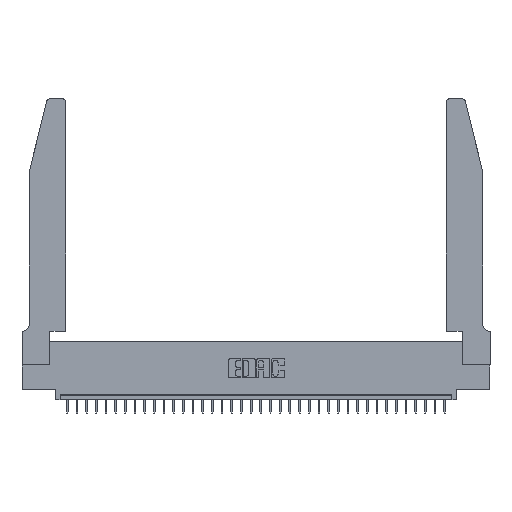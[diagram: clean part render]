
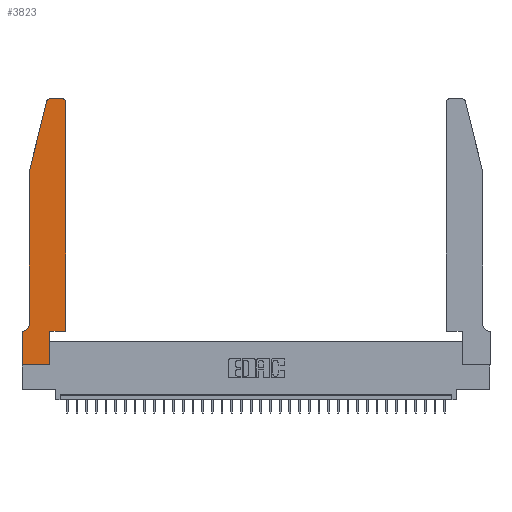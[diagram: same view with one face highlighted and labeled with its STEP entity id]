
A CAD part, top view. The second image highlights one B-rep face of the part: STEP entity #3823.
In plain terms, the highlighted planar face has unit normal (0, 0, 1).
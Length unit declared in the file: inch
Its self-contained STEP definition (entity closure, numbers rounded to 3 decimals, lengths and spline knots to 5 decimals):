
#847 = CARTESIAN_POINT ( 'NONE',  ( 0.25487, 2.72718, 0.37 ) ) ;
#1015 = ORIENTED_EDGE ( 'NONE', *, *, #24812, .T. ) ;
#1190 = ORIENTED_EDGE ( 'NONE', *, *, #3828, .T. ) ;
#1593 = DIRECTION ( 'NONE',  ( -1., 0., 0. ) ) ;
#1692 = VECTOR ( 'NONE', #20781, 39.37008 ) ;
#1829 = VERTEX_POINT ( 'NONE', #27603 ) ;
#2235 = CARTESIAN_POINT ( 'NONE',  ( 0.2865, 0., 0.37 ) ) ;
#2240 = DIRECTION ( 'NONE',  ( -0.239, -0.971, 0. ) ) ;
#2450 = CARTESIAN_POINT ( 'NONE',  ( 0.0755, 2., 0.37 ) ) ;
#3590 = LINE ( 'NONE', #11476, #9522 ) ;
#3823 = ADVANCED_FACE ( 'NONE', ( #34848 ), #24160, .T. ) ;
#3828 = EDGE_CURVE ( 'NONE', #14157, #1829, #30691, .T. ) ;
#3965 = CARTESIAN_POINT ( 'NONE',  ( 0.4505, 0.35, 0.37 ) ) ;
#4563 = VERTEX_POINT ( 'NONE', #3965 ) ;
#5346 = VERTEX_POINT ( 'NONE', #847 ) ;
#5575 = CARTESIAN_POINT ( 'NONE',  ( 0.2605, 2.75, 0.37 ) ) ;
#5810 = VERTEX_POINT ( 'NONE', #10276 ) ;
#6458 = DIRECTION ( 'NONE',  ( 0., 1., 0. ) ) ;
#6768 = CARTESIAN_POINT ( 'NONE',  ( 0., 0., 0.37 ) ) ;
#7005 = DIRECTION ( 'NONE',  ( 1., 0., 0. ) ) ;
#7046 = DIRECTION ( 'NONE',  ( 0., 0., 1. ) ) ;
#7713 = CARTESIAN_POINT ( 'NONE',  ( 0.0755, 0.42, 0.37 ) ) ;
#7977 = EDGE_CURVE ( 'NONE', #1829, #10247, #18263, .T. ) ;
#8146 = CARTESIAN_POINT ( 'NONE',  ( 0.0755, 2., 0.37 ) ) ;
#8267 = VECTOR ( 'NONE', #17427, 39.37008 ) ;
#8337 = AXIS2_PLACEMENT_3D ( 'NONE', #20620, #31492, #7005 ) ;
#8367 = AXIS2_PLACEMENT_3D ( 'NONE', #18161, #7046, #28876 ) ;
#8486 = VERTEX_POINT ( 'NONE', #14082 ) ;
#8594 = LINE ( 'NONE', #5575, #32066 ) ;
#8899 = CIRCLE ( 'NONE', #8337, 0.03 ) ;
#8989 = AXIS2_PLACEMENT_3D ( 'NONE', #20768, #29332, #15219 ) ;
#9522 = VECTOR ( 'NONE', #6458, 39.37008 ) ;
#9528 = EDGE_CURVE ( 'NONE', #17340, #18297, #35271, .T. ) ;
#9600 = EDGE_CURVE ( 'NONE', #10247, #17340, #11812, .T. ) ;
#10247 = VERTEX_POINT ( 'NONE', #26422 ) ;
#10276 = CARTESIAN_POINT ( 'NONE',  ( 0.2865, 0.35, 0.37 ) ) ;
#10323 = VERTEX_POINT ( 'NONE', #20697 ) ;
#11476 = CARTESIAN_POINT ( 'NONE',  ( 0.4505, 0.35, 0.37 ) ) ;
#11812 = LINE ( 'NONE', #6768, #25232 ) ;
#12851 = VERTEX_POINT ( 'NONE', #2450 ) ;
#12897 = DIRECTION ( 'NONE',  ( 0., 0., -1. ) ) ;
#13133 = ORIENTED_EDGE ( 'NONE', *, *, #9600, .T. ) ;
#13469 = EDGE_CURVE ( 'NONE', #12851, #14157, #15286, .T. ) ;
#13515 = ORIENTED_EDGE ( 'NONE', *, *, #29481, .T. ) ;
#14081 = VERTEX_POINT ( 'NONE', #26514 ) ;
#14082 = CARTESIAN_POINT ( 'NONE',  ( 0.284, 2.75, 0.37 ) ) ;
#14157 = VERTEX_POINT ( 'NONE', #7713 ) ;
#14248 = ORIENTED_EDGE ( 'NONE', *, *, #32844, .T. ) ;
#14506 = EDGE_CURVE ( 'NONE', #5346, #12851, #21603, .T. ) ;
#15219 = DIRECTION ( 'NONE',  ( 1., 0., 0. ) ) ;
#15286 = LINE ( 'NONE', #20478, #8267 ) ;
#15913 = ORIENTED_EDGE ( 'NONE', *, *, #13469, .T. ) ;
#15987 = CARTESIAN_POINT ( 'NONE',  ( 0., 0., 0.37 ) ) ;
#17340 = VERTEX_POINT ( 'NONE', #23679 ) ;
#17427 = DIRECTION ( 'NONE',  ( 0., -1., 0. ) ) ;
#18161 = CARTESIAN_POINT ( 'NONE',  ( 0.284, 2.72, 0.37 ) ) ;
#18263 = LINE ( 'NONE', #18621, #1692 ) ;
#18297 = VERTEX_POINT ( 'NONE', #2235 ) ;
#18302 = CARTESIAN_POINT ( 'NONE',  ( 0.2865, 0.35, 0.37 ) ) ;
#18621 = CARTESIAN_POINT ( 'NONE',  ( 0.0755, 0.35, 0.37 ) ) ;
#18953 = VECTOR ( 'NONE', #32927, 39.37008 ) ;
#19339 = LINE ( 'NONE', #30062, #31665 ) ;
#20091 = EDGE_LOOP ( 'NONE', ( #13515, #24118, #20283, #15913, #1190, #23539, #13133, #32433, #14248, #1015, #23552, #31380 ) ) ;
#20283 = ORIENTED_EDGE ( 'NONE', *, *, #14506, .T. ) ;
#20478 = CARTESIAN_POINT ( 'NONE',  ( 0.0755, 2., 0.37 ) ) ;
#20620 = CARTESIAN_POINT ( 'NONE',  ( 0.4205, 2.72, 0.37 ) ) ;
#20697 = CARTESIAN_POINT ( 'NONE',  ( 0.4505, 2.72, 0.37 ) ) ;
#20768 = CARTESIAN_POINT ( 'NONE',  ( 0., 0.35, 0.37 ) ) ;
#20781 = DIRECTION ( 'NONE',  ( -1., 0., 0. ) ) ;
#21603 = LINE ( 'NONE', #8146, #33895 ) ;
#23539 = ORIENTED_EDGE ( 'NONE', *, *, #7977, .T. ) ;
#23552 = ORIENTED_EDGE ( 'NONE', *, *, #27095, .T. ) ;
#23679 = CARTESIAN_POINT ( 'NONE',  ( 0., 0., 0.37 ) ) ;
#23816 = CIRCLE ( 'NONE', #8367, 0.03 ) ;
#24118 = ORIENTED_EDGE ( 'NONE', *, *, #27023, .T. ) ;
#24160 = PLANE ( 'NONE',  #8989 ) ;
#24812 = EDGE_CURVE ( 'NONE', #5810, #4563, #19339, .T. ) ;
#24822 = VECTOR ( 'NONE', #29201, 39.37008 ) ;
#25232 = VECTOR ( 'NONE', #33936, 39.37008 ) ;
#26148 = AXIS2_PLACEMENT_3D ( 'NONE', #34496, #12897, #1593 ) ;
#26422 = CARTESIAN_POINT ( 'NONE',  ( 0., 0.35, 0.37 ) ) ;
#26514 = CARTESIAN_POINT ( 'NONE',  ( 0.4205, 2.75, 0.37 ) ) ;
#27023 = EDGE_CURVE ( 'NONE', #8486, #5346, #23816, .T. ) ;
#27095 = EDGE_CURVE ( 'NONE', #4563, #10323, #3590, .T. ) ;
#27551 = DIRECTION ( 'NONE',  ( 1., 0., 0. ) ) ;
#27603 = CARTESIAN_POINT ( 'NONE',  ( 0.0055, 0.35, 0.37 ) ) ;
#28096 = EDGE_CURVE ( 'NONE', #10323, #14081, #8899, .T. ) ;
#28876 = DIRECTION ( 'NONE',  ( 1., 0., 0. ) ) ;
#29201 = DIRECTION ( 'NONE',  ( 0., 1., 0. ) ) ;
#29332 = DIRECTION ( 'NONE',  ( 0., 0., 1. ) ) ;
#29481 = EDGE_CURVE ( 'NONE', #14081, #8486, #8594, .T. ) ;
#30062 = CARTESIAN_POINT ( 'NONE',  ( 0.4505, 0.35, 0.37 ) ) ;
#30691 = CIRCLE ( 'NONE', #26148, 0.07 ) ;
#31380 = ORIENTED_EDGE ( 'NONE', *, *, #28096, .T. ) ;
#31492 = DIRECTION ( 'NONE',  ( 0., 0., 1. ) ) ;
#31665 = VECTOR ( 'NONE', #27551, 39.37008 ) ;
#31877 = LINE ( 'NONE', #18302, #24822 ) ;
#32066 = VECTOR ( 'NONE', #35256, 39.37008 ) ;
#32433 = ORIENTED_EDGE ( 'NONE', *, *, #9528, .T. ) ;
#32844 = EDGE_CURVE ( 'NONE', #18297, #5810, #31877, .T. ) ;
#32927 = DIRECTION ( 'NONE',  ( 1., 0., 0. ) ) ;
#33895 = VECTOR ( 'NONE', #2240, 39.37008 ) ;
#33936 = DIRECTION ( 'NONE',  ( 0., -1., 0. ) ) ;
#34496 = CARTESIAN_POINT ( 'NONE',  ( 0.0055, 0.42, 0.37 ) ) ;
#34848 = FACE_OUTER_BOUND ( 'NONE', #20091, .T. ) ;
#35256 = DIRECTION ( 'NONE',  ( -1., 0., 0. ) ) ;
#35271 = LINE ( 'NONE', #15987, #18953 ) ;
